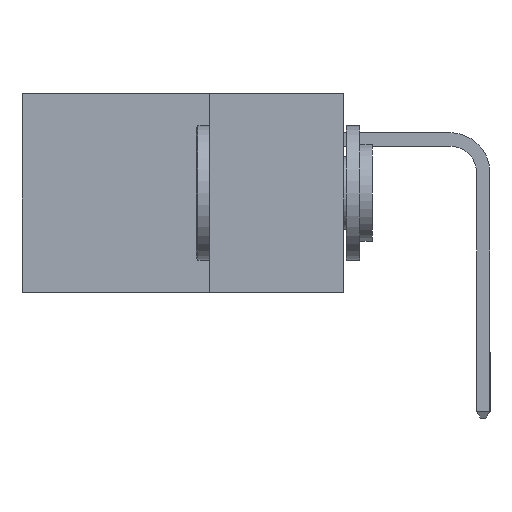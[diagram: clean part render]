
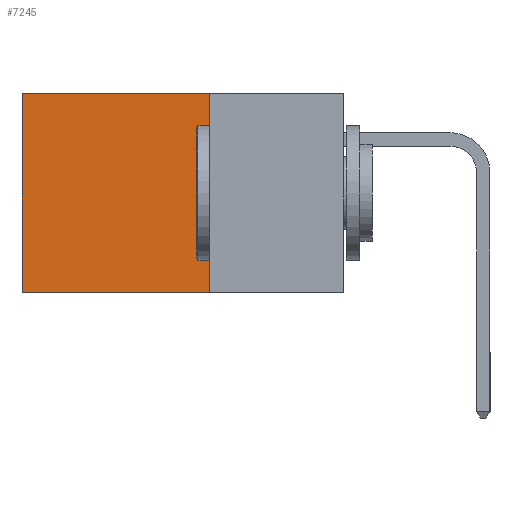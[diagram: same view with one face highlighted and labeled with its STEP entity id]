
A CAD part, left-side view. The second image highlights one B-rep face of the part: STEP entity #7245.
In plain terms, the highlighted planar face has unit normal (-1, 0, 0).
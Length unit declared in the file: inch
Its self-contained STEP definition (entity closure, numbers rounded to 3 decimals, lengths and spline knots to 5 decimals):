
#13 = DIRECTION ( 'NONE',  ( 0., 0., -1. ) ) ;
#156 = CARTESIAN_POINT ( 'NONE',  ( 0.298, 0.25, 0. ) ) ;
#459 = VERTEX_POINT ( 'NONE', #10260 ) ;
#1070 = VECTOR ( 'NONE', #5936, 39.37008 ) ;
#1850 = VECTOR ( 'NONE', #10680, 39.37008 ) ;
#1906 = VERTEX_POINT ( 'NONE', #2876 ) ;
#2876 = CARTESIAN_POINT ( 'NONE',  ( 0.298, 0.25, -0.37 ) ) ;
#3610 = ORIENTED_EDGE ( 'NONE', *, *, #12520, .T. ) ;
#4148 = LINE ( 'NONE', #6052, #1070 ) ;
#4161 = EDGE_CURVE ( 'NONE', #6554, #1906, #8090, .T. ) ;
#4386 = CARTESIAN_POINT ( 'NONE',  ( 0.298, 0.25, 0. ) ) ;
#4653 = DIRECTION ( 'NONE',  ( 0., 1., 0. ) ) ;
#5034 = AXIS2_PLACEMENT_3D ( 'NONE', #156, #12727, #8619 ) ;
#5267 = CARTESIAN_POINT ( 'NONE',  ( 0.298, 0.25, 0. ) ) ;
#5547 = CARTESIAN_POINT ( 'NONE',  ( 0.298, 0.25, 0. ) ) ;
#5692 = ORIENTED_EDGE ( 'NONE', *, *, #8659, .T. ) ;
#5936 = DIRECTION ( 'NONE',  ( 0., 0., -1. ) ) ;
#6052 = CARTESIAN_POINT ( 'NONE',  ( 0.298, 0.6, 0. ) ) ;
#6384 = VERTEX_POINT ( 'NONE', #8477 ) ;
#6471 = EDGE_CURVE ( 'NONE', #1906, #459, #7759, .T. ) ;
#6554 = VERTEX_POINT ( 'NONE', #4386 ) ;
#7245 = ADVANCED_FACE ( 'NONE', ( #8885 ), #11615, .F. ) ;
#7759 = LINE ( 'NONE', #9788, #1850 ) ;
#8090 = LINE ( 'NONE', #5267, #9921 ) ;
#8330 = ORIENTED_EDGE ( 'NONE', *, *, #6471, .F. ) ;
#8477 = CARTESIAN_POINT ( 'NONE',  ( 0.298, 0.6, 0. ) ) ;
#8619 = DIRECTION ( 'NONE',  ( 0., 0., -1. ) ) ;
#8659 = EDGE_CURVE ( 'NONE', #6384, #459, #4148, .T. ) ;
#8807 = LINE ( 'NONE', #5547, #10602 ) ;
#8885 = FACE_OUTER_BOUND ( 'NONE', #9455, .T. ) ;
#9455 = EDGE_LOOP ( 'NONE', ( #5692, #8330, #9901, #3610 ) ) ;
#9788 = CARTESIAN_POINT ( 'NONE',  ( 0.298, 0.25, -0.37 ) ) ;
#9901 = ORIENTED_EDGE ( 'NONE', *, *, #4161, .F. ) ;
#9921 = VECTOR ( 'NONE', #13, 39.37008 ) ;
#10260 = CARTESIAN_POINT ( 'NONE',  ( 0.298, 0.6, -0.37 ) ) ;
#10602 = VECTOR ( 'NONE', #4653, 39.37008 ) ;
#10680 = DIRECTION ( 'NONE',  ( 0., 1., 0. ) ) ;
#11615 = PLANE ( 'NONE',  #5034 ) ;
#12520 = EDGE_CURVE ( 'NONE', #6554, #6384, #8807, .T. ) ;
#12727 = DIRECTION ( 'NONE',  ( 1., 0., 0. ) ) ;
